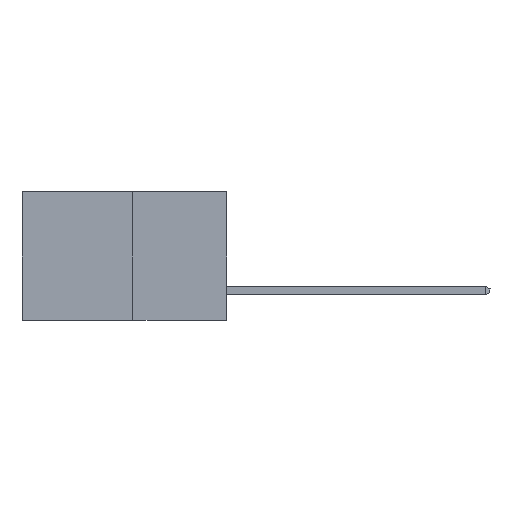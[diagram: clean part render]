
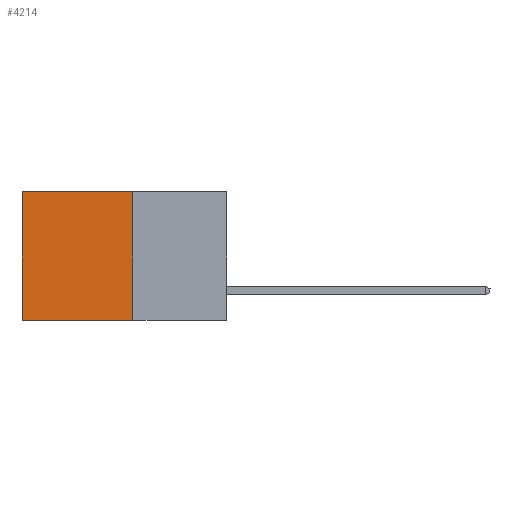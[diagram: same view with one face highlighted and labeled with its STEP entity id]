
A CAD part, left-side view. The second image highlights one B-rep face of the part: STEP entity #4214.
In plain terms, the highlighted planar face has unit normal (-1, 0, 0).
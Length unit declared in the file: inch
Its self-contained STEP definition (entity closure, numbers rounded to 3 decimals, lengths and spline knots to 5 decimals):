
#913 = DIRECTION ( 'NONE',  ( 0., 0., -1. ) ) ;
#1356 = DIRECTION ( 'NONE',  ( 0., 1., 0. ) ) ;
#1596 = VERTEX_POINT ( 'NONE', #5689 ) ;
#2413 = VECTOR ( 'NONE', #11930, 39.37008 ) ;
#2781 = ORIENTED_EDGE ( 'NONE', *, *, #13212, .F. ) ;
#2988 = ORIENTED_EDGE ( 'NONE', *, *, #12463, .T. ) ;
#3928 = CARTESIAN_POINT ( 'NONE',  ( 0.277, 0.27, 0. ) ) ;
#4214 = ADVANCED_FACE ( 'NONE', ( #9467 ), #12055, .F. ) ;
#4354 = LINE ( 'NONE', #15799, #13807 ) ;
#4386 = EDGE_LOOP ( 'NONE', ( #10686, #2781, #10521, #2988 ) ) ;
#4404 = AXIS2_PLACEMENT_3D ( 'NONE', #11895, #11782, #11805 ) ;
#5448 = LINE ( 'NONE', #8909, #11935 ) ;
#5487 = VERTEX_POINT ( 'NONE', #7423 ) ;
#5579 = VERTEX_POINT ( 'NONE', #6755 ) ;
#5689 = CARTESIAN_POINT ( 'NONE',  ( 0.277, 0.27, -0.37 ) ) ;
#5821 = CARTESIAN_POINT ( 'NONE',  ( 0.277, 0.59, -0.37 ) ) ;
#5824 = LINE ( 'NONE', #5821, #2413 ) ;
#6490 = LINE ( 'NONE', #3928, #9678 ) ;
#6755 = CARTESIAN_POINT ( 'NONE',  ( 0.277, 0.59, 0. ) ) ;
#7423 = CARTESIAN_POINT ( 'NONE',  ( 0.277, 0.27, 0. ) ) ;
#8388 = CARTESIAN_POINT ( 'NONE',  ( 0.277, 0.59, -0.37 ) ) ;
#8909 = CARTESIAN_POINT ( 'NONE',  ( 0.277, 0.27, -0.37 ) ) ;
#9326 = VERTEX_POINT ( 'NONE', #8388 ) ;
#9467 = FACE_OUTER_BOUND ( 'NONE', #4386, .T. ) ;
#9678 = VECTOR ( 'NONE', #11339, 39.37008 ) ;
#10521 = ORIENTED_EDGE ( 'NONE', *, *, #16131, .F. ) ;
#10686 = ORIENTED_EDGE ( 'NONE', *, *, #14053, .T. ) ;
#11339 = DIRECTION ( 'NONE',  ( 0., 1., 0. ) ) ;
#11782 = DIRECTION ( 'NONE',  ( 1., 0., 0. ) ) ;
#11805 = DIRECTION ( 'NONE',  ( 0., 0., -1. ) ) ;
#11895 = CARTESIAN_POINT ( 'NONE',  ( 0.277, 0.27, -0.37 ) ) ;
#11930 = DIRECTION ( 'NONE',  ( 0., 0., -1. ) ) ;
#11935 = VECTOR ( 'NONE', #1356, 39.37008 ) ;
#12055 = PLANE ( 'NONE',  #4404 ) ;
#12463 = EDGE_CURVE ( 'NONE', #5487, #5579, #6490, .T. ) ;
#13212 = EDGE_CURVE ( 'NONE', #1596, #9326, #5448, .T. ) ;
#13807 = VECTOR ( 'NONE', #913, 39.37008 ) ;
#14053 = EDGE_CURVE ( 'NONE', #5579, #9326, #5824, .T. ) ;
#15799 = CARTESIAN_POINT ( 'NONE',  ( 0.277, 0.27, -0.37 ) ) ;
#16131 = EDGE_CURVE ( 'NONE', #5487, #1596, #4354, .T. ) ;
